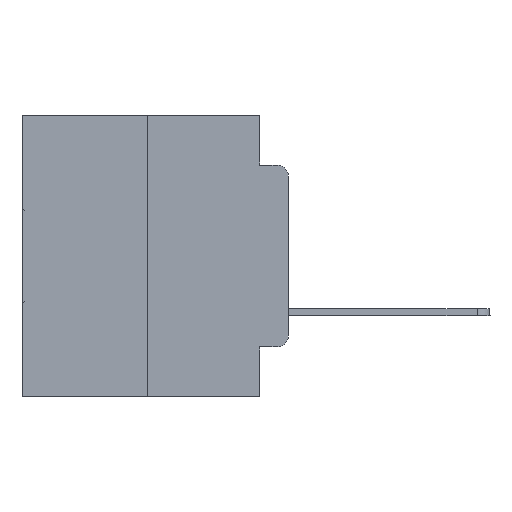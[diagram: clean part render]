
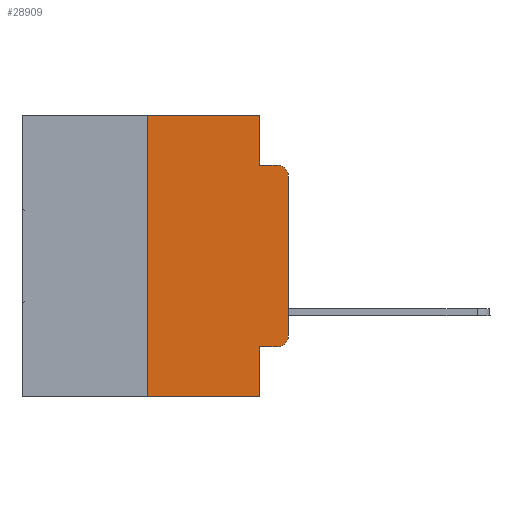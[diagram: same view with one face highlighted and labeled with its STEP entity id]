
A CAD part, left-side view. The second image highlights one B-rep face of the part: STEP entity #28909.
In plain terms, the highlighted planar face has unit normal (-1, 0, 0).
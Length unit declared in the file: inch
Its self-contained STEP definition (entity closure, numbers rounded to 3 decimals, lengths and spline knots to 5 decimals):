
#51 = VECTOR ( 'NONE', #2247, 39.37008 ) ;
#91 = CARTESIAN_POINT ( 'NONE',  ( 0., 0.02, -0.3915 ) ) ;
#314 = CARTESIAN_POINT ( 'NONE',  ( 0., 0.051, -0.4115 ) ) ;
#967 = LINE ( 'NONE', #13345, #19138 ) ;
#1271 = AXIS2_PLACEMENT_3D ( 'NONE', #91, #2515, #9802 ) ;
#1827 = VERTEX_POINT ( 'NONE', #23772 ) ;
#1954 = ORIENTED_EDGE ( 'NONE', *, *, #8572, .T. ) ;
#2247 = DIRECTION ( 'NONE',  ( 0., 0., 1. ) ) ;
#2515 = DIRECTION ( 'NONE',  ( -1., 0., 0. ) ) ;
#2517 = EDGE_LOOP ( 'NONE', ( #10418, #17261, #13812, #18675, #23527, #18997, #7374, #11738, #1954, #27974 ) ) ;
#2941 = CIRCLE ( 'NONE', #1271, 0.02 ) ;
#3410 = VECTOR ( 'NONE', #6042, 39.37008 ) ;
#3470 = CARTESIAN_POINT ( 'NONE',  ( 0., 0.473, 0. ) ) ;
#3799 = VERTEX_POINT ( 'NONE', #30316 ) ;
#5186 = EDGE_CURVE ( 'NONE', #26701, #28333, #13118, .T. ) ;
#5341 = CARTESIAN_POINT ( 'NONE',  ( 0., 0.02, -0.4115 ) ) ;
#6042 = DIRECTION ( 'NONE',  ( 0., 0., -1. ) ) ;
#6101 = DIRECTION ( 'NONE',  ( 0., -1., 0. ) ) ;
#6371 = CARTESIAN_POINT ( 'NONE',  ( 0., 0.051, 0. ) ) ;
#6697 = DIRECTION ( 'NONE',  ( 0., -1., 0. ) ) ;
#6928 = DIRECTION ( 'NONE',  ( 0., 0., -1. ) ) ;
#7028 = AXIS2_PLACEMENT_3D ( 'NONE', #18632, #23883, #9428 ) ;
#7232 = LINE ( 'NONE', #23903, #51 ) ;
#7357 = FACE_OUTER_BOUND ( 'NONE', #2517, .T. ) ;
#7374 = ORIENTED_EDGE ( 'NONE', *, *, #5186, .T. ) ;
#7847 = LINE ( 'NONE', #11214, #26393 ) ;
#8572 = EDGE_CURVE ( 'NONE', #18295, #18702, #26092, .T. ) ;
#8704 = LINE ( 'NONE', #3470, #10169 ) ;
#8991 = CARTESIAN_POINT ( 'NONE',  ( 0., 0.25, -0.5 ) ) ;
#9428 = DIRECTION ( 'NONE',  ( 0., 0., -1. ) ) ;
#9469 = CARTESIAN_POINT ( 'NONE',  ( 0., 0.02, -0.1085 ) ) ;
#9802 = DIRECTION ( 'NONE',  ( 0., 0., -1. ) ) ;
#10025 = VECTOR ( 'NONE', #6697, 39.37008 ) ;
#10169 = VECTOR ( 'NONE', #6101, 39.37008 ) ;
#10418 = ORIENTED_EDGE ( 'NONE', *, *, #30932, .T. ) ;
#10999 = CARTESIAN_POINT ( 'NONE',  ( 0., 0.051, 0. ) ) ;
#11092 = VECTOR ( 'NONE', #13162, 39.37008 ) ;
#11214 = CARTESIAN_POINT ( 'NONE',  ( 0., 0.051, 0. ) ) ;
#11738 = ORIENTED_EDGE ( 'NONE', *, *, #22416, .F. ) ;
#12299 = DIRECTION ( 'NONE',  ( 0., -1., 0. ) ) ;
#13117 = CARTESIAN_POINT ( 'NONE',  ( 0., 0.473, -0.5 ) ) ;
#13118 = LINE ( 'NONE', #13117, #10025 ) ;
#13162 = DIRECTION ( 'NONE',  ( 0., -1., 0. ) ) ;
#13345 = CARTESIAN_POINT ( 'NONE',  ( 0., 0.25, 0. ) ) ;
#13382 = VERTEX_POINT ( 'NONE', #10999 ) ;
#13812 = ORIENTED_EDGE ( 'NONE', *, *, #25014, .F. ) ;
#13976 = CARTESIAN_POINT ( 'NONE',  ( 0., 0.051, -0.4115 ) ) ;
#14166 = VERTEX_POINT ( 'NONE', #24506 ) ;
#15970 = DIRECTION ( 'NONE',  ( 0., 0., -1. ) ) ;
#17261 = ORIENTED_EDGE ( 'NONE', *, *, #24722, .T. ) ;
#17936 = EDGE_CURVE ( 'NONE', #13382, #19579, #25355, .T. ) ;
#18295 = VERTEX_POINT ( 'NONE', #13976 ) ;
#18309 = PLANE ( 'NONE',  #7028 ) ;
#18632 = CARTESIAN_POINT ( 'NONE',  ( 0., 0.473, 0. ) ) ;
#18675 = ORIENTED_EDGE ( 'NONE', *, *, #17936, .F. ) ;
#18702 = VERTEX_POINT ( 'NONE', #5341 ) ;
#18997 = ORIENTED_EDGE ( 'NONE', *, *, #23454, .F. ) ;
#19138 = VECTOR ( 'NONE', #27970, 39.37008 ) ;
#19501 = EDGE_CURVE ( 'NONE', #14166, #13382, #8704, .T. ) ;
#19579 = VERTEX_POINT ( 'NONE', #28148 ) ;
#19593 = VECTOR ( 'NONE', #12299, 39.37008 ) ;
#20451 = LINE ( 'NONE', #29545, #11092 ) ;
#22416 = EDGE_CURVE ( 'NONE', #18295, #28333, #7847, .T. ) ;
#23454 = EDGE_CURVE ( 'NONE', #26701, #14166, #967, .T. ) ;
#23527 = ORIENTED_EDGE ( 'NONE', *, *, #19501, .F. ) ;
#23584 = CARTESIAN_POINT ( 'NONE',  ( 0., 0.051, -0.5 ) ) ;
#23772 = CARTESIAN_POINT ( 'NONE',  ( 0., 0., -0.1085 ) ) ;
#23883 = DIRECTION ( 'NONE',  ( 1., 0., 0. ) ) ;
#23903 = CARTESIAN_POINT ( 'NONE',  ( 0., 0., 0. ) ) ;
#23905 = AXIS2_PLACEMENT_3D ( 'NONE', #9469, #24033, #6928 ) ;
#24033 = DIRECTION ( 'NONE',  ( -1., 0., 0. ) ) ;
#24506 = CARTESIAN_POINT ( 'NONE',  ( 0., 0.25, 0. ) ) ;
#24722 = EDGE_CURVE ( 'NONE', #1827, #26643, #25030, .T. ) ;
#25014 = EDGE_CURVE ( 'NONE', #19579, #26643, #20451, .T. ) ;
#25030 = CIRCLE ( 'NONE', #23905, 0.02 ) ;
#25355 = LINE ( 'NONE', #6371, #3410 ) ;
#26092 = LINE ( 'NONE', #314, #19593 ) ;
#26318 = EDGE_CURVE ( 'NONE', #18702, #3799, #2941, .T. ) ;
#26393 = VECTOR ( 'NONE', #15970, 39.37008 ) ;
#26643 = VERTEX_POINT ( 'NONE', #30173 ) ;
#26701 = VERTEX_POINT ( 'NONE', #8991 ) ;
#27970 = DIRECTION ( 'NONE',  ( 0., 0., 1. ) ) ;
#27974 = ORIENTED_EDGE ( 'NONE', *, *, #26318, .T. ) ;
#28148 = CARTESIAN_POINT ( 'NONE',  ( 0., 0.051, -0.0885 ) ) ;
#28333 = VERTEX_POINT ( 'NONE', #23584 ) ;
#28909 = ADVANCED_FACE ( 'NONE', ( #7357 ), #18309, .F. ) ;
#29545 = CARTESIAN_POINT ( 'NONE',  ( 0., 0.051, -0.0885 ) ) ;
#30173 = CARTESIAN_POINT ( 'NONE',  ( 0., 0.02, -0.0885 ) ) ;
#30316 = CARTESIAN_POINT ( 'NONE',  ( 0., 0., -0.3915 ) ) ;
#30932 = EDGE_CURVE ( 'NONE', #3799, #1827, #7232, .T. ) ;
